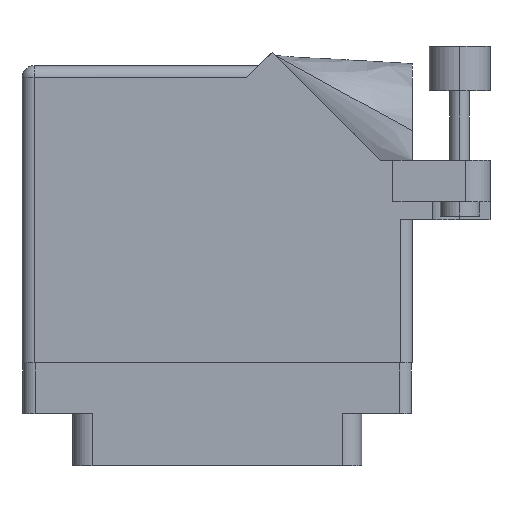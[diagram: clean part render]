
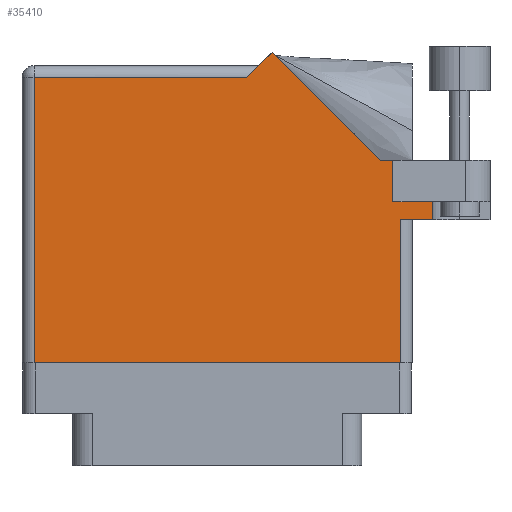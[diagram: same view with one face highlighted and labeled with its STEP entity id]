
A CAD part, front view. The second image highlights one B-rep face of the part: STEP entity #35410.
In plain terms, the highlighted face is planar.
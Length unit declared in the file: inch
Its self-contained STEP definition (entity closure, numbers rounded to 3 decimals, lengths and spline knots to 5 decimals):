
#446 = CARTESIAN_POINT ( 'NONE',  ( 2.1115, 1.16177, 0. ) ) ;
#718 = CARTESIAN_POINT ( 'NONE',  ( 2.1115, 0.737, 0. ) ) ;
#781 = ORIENTED_EDGE ( 'NONE', *, *, #10153, .T. ) ;
#797 = VECTOR ( 'NONE', #28531, 39.37008 ) ;
#1210 = DIRECTION ( 'NONE',  ( 0., 1., 0. ) ) ;
#1709 = PLANE ( 'NONE',  #24901 ) ;
#2181 = CARTESIAN_POINT ( 'NONE',  ( 0.062, 1.468, 0. ) ) ;
#2600 = CARTESIAN_POINT ( 'NONE',  ( 0.062, 0., 0. ) ) ;
#3590 = CARTESIAN_POINT ( 'NONE',  ( 1.155, 1.468, 0. ) ) ;
#3822 = VERTEX_POINT ( 'NONE', #25893 ) ;
#4344 = CARTESIAN_POINT ( 'NONE',  ( 0., 1.468, 0. ) ) ;
#4638 = CARTESIAN_POINT ( 'NONE',  ( 1.28771, 1.60071, 0. ) ) ;
#4866 = ORIENTED_EDGE ( 'NONE', *, *, #11425, .T. ) ;
#5977 = VECTOR ( 'NONE', #30596, 39.37008 ) ;
#5997 = EDGE_CURVE ( 'NONE', #29487, #31753, #15026, .T. ) ;
#6202 = DIRECTION ( 'NONE',  ( -0.707, 0.707, 0. ) ) ;
#7994 = VECTOR ( 'NONE', #30403, 39.37008 ) ;
#8040 = EDGE_CURVE ( 'NONE', #23918, #35277, #26305, .T. ) ;
#8712 = VECTOR ( 'NONE', #1210, 39.37008 ) ;
#9588 = ORIENTED_EDGE ( 'NONE', *, *, #8040, .T. ) ;
#10153 = EDGE_CURVE ( 'NONE', #39275, #26165, #20227, .T. ) ;
#10178 = VERTEX_POINT ( 'NONE', #10667 ) ;
#10667 = CARTESIAN_POINT ( 'NONE',  ( 1.948, 0.737, 0. ) ) ;
#11064 = CARTESIAN_POINT ( 'NONE',  ( 2.41, 1.044, 0. ) ) ;
#11425 = EDGE_CURVE ( 'NONE', #10178, #33427, #32450, .T. ) ;
#11564 = EDGE_CURVE ( 'NONE', #3822, #39275, #32936, .T. ) ;
#11612 = ORIENTED_EDGE ( 'NONE', *, *, #19380, .T. ) ;
#11696 = LINE ( 'NONE', #21413, #5977 ) ;
#12481 = VECTOR ( 'NONE', #18877, 39.37008 ) ;
#12754 = LINE ( 'NONE', #33955, #25113 ) ;
#13498 = CARTESIAN_POINT ( 'NONE',  ( 2.1115, 0.831, 0. ) ) ;
#13869 = CARTESIAN_POINT ( 'NONE',  ( 1.91, 1.044, 0. ) ) ;
#14206 = ORIENTED_EDGE ( 'NONE', *, *, #20599, .T. ) ;
#14810 = DIRECTION ( 'NONE',  ( 1., 0., 0. ) ) ;
#15016 = VECTOR ( 'NONE', #28846, 39.37008 ) ;
#15026 = LINE ( 'NONE', #4344, #797 ) ;
#16301 = CARTESIAN_POINT ( 'NONE',  ( 1.91, 0.831, 0. ) ) ;
#16683 = DIRECTION ( 'NONE',  ( -0.707, -0.707, 0. ) ) ;
#16786 = ORIENTED_EDGE ( 'NONE', *, *, #25600, .F. ) ;
#17435 = ORIENTED_EDGE ( 'NONE', *, *, #32024, .T. ) ;
#18537 = CARTESIAN_POINT ( 'NONE',  ( 2.01, 0.737, 0. ) ) ;
#18673 = DIRECTION ( 'NONE',  ( 1., 0., 0. ) ) ;
#18877 = DIRECTION ( 'NONE',  ( 1., 0., 0. ) ) ;
#18908 = CARTESIAN_POINT ( 'NONE',  ( 1.948, 0., 0. ) ) ;
#19214 = ORIENTED_EDGE ( 'NONE', *, *, #11564, .T. ) ;
#19380 = EDGE_CURVE ( 'NONE', #30271, #29487, #30921, .T. ) ;
#19977 = DIRECTION ( 'NONE',  ( 0., 0., -1. ) ) ;
#20227 = LINE ( 'NONE', #11064, #15016 ) ;
#20599 = EDGE_CURVE ( 'NONE', #31753, #23918, #12754, .T. ) ;
#21413 = CARTESIAN_POINT ( 'NONE',  ( 1.948, 0.737, 0. ) ) ;
#21901 = CARTESIAN_POINT ( 'NONE',  ( 1.84442, 1.044, 0. ) ) ;
#22103 = CARTESIAN_POINT ( 'NONE',  ( 0., 0., 0. ) ) ;
#22600 = DIRECTION ( 'NONE',  ( 0., -1., 0. ) ) ;
#22833 = VECTOR ( 'NONE', #16683, 39.37008 ) ;
#23653 = CARTESIAN_POINT ( 'NONE',  ( 1.84442, 1.044, 0. ) ) ;
#23918 = VERTEX_POINT ( 'NONE', #2600 ) ;
#24901 = AXIS2_PLACEMENT_3D ( 'NONE', #32066, #19977, #26231 ) ;
#25113 = VECTOR ( 'NONE', #22600, 39.37008 ) ;
#25305 = LINE ( 'NONE', #21901, #34301 ) ;
#25600 = EDGE_CURVE ( 'NONE', #3822, #37029, #30936, .T. ) ;
#25847 = CARTESIAN_POINT ( 'NONE',  ( 1.217, 1.53, 0. ) ) ;
#25893 = CARTESIAN_POINT ( 'NONE',  ( 1.91, 0.831, 0. ) ) ;
#25911 = EDGE_LOOP ( 'NONE', ( #9588, #31951, #4866, #35841, #16786, #19214, #781, #17435, #11612, #38725, #14206 ) ) ;
#26165 = VERTEX_POINT ( 'NONE', #23653 ) ;
#26231 = DIRECTION ( 'NONE',  ( -1., 0., 0. ) ) ;
#26305 = LINE ( 'NONE', #22103, #12481 ) ;
#26863 = EDGE_CURVE ( 'NONE', #37029, #33427, #36038, .T. ) ;
#28060 = VECTOR ( 'NONE', #14810, 39.37008 ) ;
#28531 = DIRECTION ( 'NONE',  ( -1., 0., 0. ) ) ;
#28846 = DIRECTION ( 'NONE',  ( -1., 0., 0. ) ) ;
#29148 = VECTOR ( 'NONE', #18673, 39.37008 ) ;
#29487 = VERTEX_POINT ( 'NONE', #3590 ) ;
#30010 = EDGE_CURVE ( 'NONE', #35277, #10178, #11696, .T. ) ;
#30271 = VERTEX_POINT ( 'NONE', #4638 ) ;
#30403 = DIRECTION ( 'NONE',  ( 0., -1., 0. ) ) ;
#30596 = DIRECTION ( 'NONE',  ( 0., 1., 0. ) ) ;
#30921 = LINE ( 'NONE', #25847, #22833 ) ;
#30936 = LINE ( 'NONE', #39113, #28060 ) ;
#31302 = FACE_OUTER_BOUND ( 'NONE', #25911, .T. ) ;
#31753 = VERTEX_POINT ( 'NONE', #2181 ) ;
#31951 = ORIENTED_EDGE ( 'NONE', *, *, #30010, .T. ) ;
#32024 = EDGE_CURVE ( 'NONE', #26165, #30271, #25305, .T. ) ;
#32066 = CARTESIAN_POINT ( 'NONE',  ( 0., 1.53, 0. ) ) ;
#32450 = LINE ( 'NONE', #18537, #29148 ) ;
#32936 = LINE ( 'NONE', #16301, #8712 ) ;
#33427 = VERTEX_POINT ( 'NONE', #718 ) ;
#33955 = CARTESIAN_POINT ( 'NONE',  ( 0.062, 0., 0. ) ) ;
#34301 = VECTOR ( 'NONE', #6202, 39.37008 ) ;
#35277 = VERTEX_POINT ( 'NONE', #18908 ) ;
#35410 = ADVANCED_FACE ( 'NONE', ( #31302 ), #1709, .F. ) ;
#35841 = ORIENTED_EDGE ( 'NONE', *, *, #26863, .F. ) ;
#36038 = LINE ( 'NONE', #446, #7994 ) ;
#37029 = VERTEX_POINT ( 'NONE', #13498 ) ;
#38725 = ORIENTED_EDGE ( 'NONE', *, *, #5997, .T. ) ;
#39113 = CARTESIAN_POINT ( 'NONE',  ( 1.91, 0.831, 0. ) ) ;
#39275 = VERTEX_POINT ( 'NONE', #13869 ) ;
